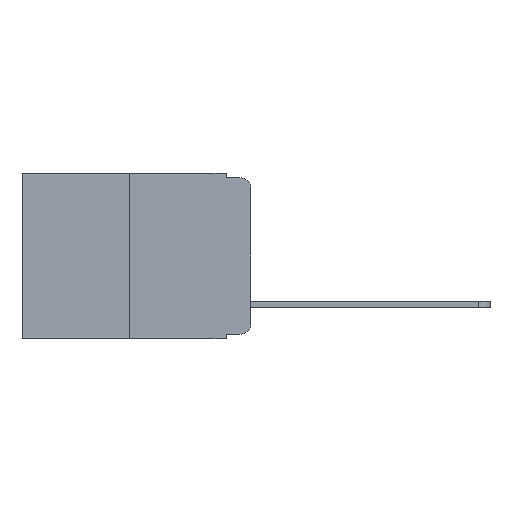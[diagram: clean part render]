
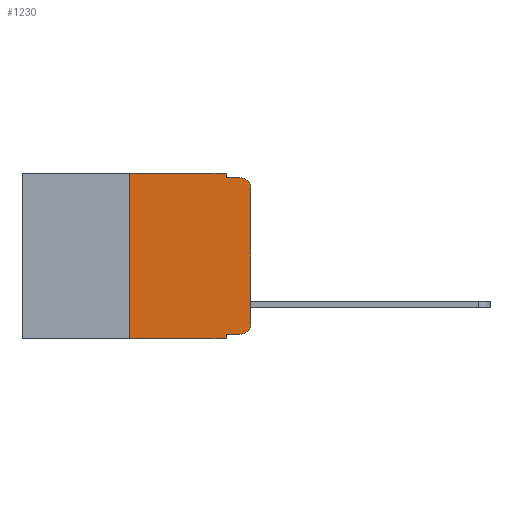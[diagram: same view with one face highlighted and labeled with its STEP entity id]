
A CAD part, left-side view. The second image highlights one B-rep face of the part: STEP entity #1230.
In plain terms, the highlighted planar face has unit normal (-1, 0, 0).
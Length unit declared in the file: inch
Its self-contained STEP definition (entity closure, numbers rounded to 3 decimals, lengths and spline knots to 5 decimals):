
#204 = CIRCLE ( 'NONE', #12012, 0.02 ) ;
#781 = CARTESIAN_POINT ( 'NONE',  ( 0., 0.02, -0.333 ) ) ;
#887 = CARTESIAN_POINT ( 'NONE',  ( 0., 0.25, 0. ) ) ;
#1215 = ORIENTED_EDGE ( 'NONE', *, *, #23683, .T. ) ;
#1230 = ADVANCED_FACE ( 'NONE', ( #8521 ), #20742, .F. ) ;
#2332 = DIRECTION ( 'NONE',  ( 0., 0., -1. ) ) ;
#2346 = VECTOR ( 'NONE', #14218, 39.37008 ) ;
#2682 = CARTESIAN_POINT ( 'NONE',  ( 0., 0.051, 0. ) ) ;
#2750 = EDGE_LOOP ( 'NONE', ( #22000, #1215, #9714, #23179, #7960, #5923, #19420, #9176, #12704, #6830 ) ) ;
#2857 = VECTOR ( 'NONE', #24087, 39.37008 ) ;
#2956 = CARTESIAN_POINT ( 'NONE',  ( 0., 0.02, -0.01 ) ) ;
#3386 = VERTEX_POINT ( 'NONE', #12868 ) ;
#3458 = EDGE_CURVE ( 'NONE', #11988, #9222, #12223, .T. ) ;
#3944 = VERTEX_POINT ( 'NONE', #2956 ) ;
#4273 = CIRCLE ( 'NONE', #19153, 0.02 ) ;
#4627 = DIRECTION ( 'NONE',  ( 0., -1., 0. ) ) ;
#4628 = DIRECTION ( 'NONE',  ( 0., -1., 0. ) ) ;
#4847 = CARTESIAN_POINT ( 'NONE',  ( 0., 0.051, -0.01 ) ) ;
#5865 = CARTESIAN_POINT ( 'NONE',  ( 0., 0.02, -0.03 ) ) ;
#5923 = ORIENTED_EDGE ( 'NONE', *, *, #20074, .F. ) ;
#5955 = CARTESIAN_POINT ( 'NONE',  ( 0., 0.25, -0.343 ) ) ;
#6243 = VERTEX_POINT ( 'NONE', #7693 ) ;
#6281 = CARTESIAN_POINT ( 'NONE',  ( 0., 0., 0. ) ) ;
#6377 = VECTOR ( 'NONE', #4628, 39.37008 ) ;
#6830 = ORIENTED_EDGE ( 'NONE', *, *, #18515, .T. ) ;
#7059 = CARTESIAN_POINT ( 'NONE',  ( 0., 0.051, -0.01 ) ) ;
#7323 = LINE ( 'NONE', #19862, #2346 ) ;
#7523 = EDGE_CURVE ( 'NONE', #9537, #10776, #7323, .T. ) ;
#7693 = CARTESIAN_POINT ( 'NONE',  ( 0., 0., -0.03 ) ) ;
#7742 = DIRECTION ( 'NONE',  ( 0., 0., -1. ) ) ;
#7840 = EDGE_CURVE ( 'NONE', #9222, #22808, #19616, .T. ) ;
#7960 = ORIENTED_EDGE ( 'NONE', *, *, #3458, .F. ) ;
#7983 = EDGE_CURVE ( 'NONE', #9537, #17198, #12288, .T. ) ;
#8521 = FACE_OUTER_BOUND ( 'NONE', #2750, .T. ) ;
#9056 = VERTEX_POINT ( 'NONE', #5955 ) ;
#9136 = CARTESIAN_POINT ( 'NONE',  ( 0., 0.051, -0.333 ) ) ;
#9176 = ORIENTED_EDGE ( 'NONE', *, *, #7523, .F. ) ;
#9222 = VERTEX_POINT ( 'NONE', #2682 ) ;
#9537 = VERTEX_POINT ( 'NONE', #9136 ) ;
#9655 = AXIS2_PLACEMENT_3D ( 'NONE', #11966, #18676, #13009 ) ;
#9714 = ORIENTED_EDGE ( 'NONE', *, *, #17434, .F. ) ;
#10776 = VERTEX_POINT ( 'NONE', #15697 ) ;
#10803 = CARTESIAN_POINT ( 'NONE',  ( 0., 0.02, -0.313 ) ) ;
#11193 = CARTESIAN_POINT ( 'NONE',  ( 0., 0.25, 0. ) ) ;
#11692 = LINE ( 'NONE', #7059, #13737 ) ;
#11705 = VECTOR ( 'NONE', #4627, 39.37008 ) ;
#11935 = EDGE_CURVE ( 'NONE', #3386, #6243, #17278, .T. ) ;
#11966 = CARTESIAN_POINT ( 'NONE',  ( 0., 0.473, 0. ) ) ;
#11988 = VERTEX_POINT ( 'NONE', #887 ) ;
#12012 = AXIS2_PLACEMENT_3D ( 'NONE', #10803, #23873, #12679 ) ;
#12223 = LINE ( 'NONE', #12339, #2857 ) ;
#12288 = LINE ( 'NONE', #17721, #11705 ) ;
#12339 = CARTESIAN_POINT ( 'NONE',  ( 0., 0.473, 0. ) ) ;
#12597 = EDGE_CURVE ( 'NONE', #9056, #10776, #16949, .T. ) ;
#12679 = DIRECTION ( 'NONE',  ( 0., 0., -1. ) ) ;
#12704 = ORIENTED_EDGE ( 'NONE', *, *, #7983, .T. ) ;
#12868 = CARTESIAN_POINT ( 'NONE',  ( 0., 0., -0.313 ) ) ;
#13009 = DIRECTION ( 'NONE',  ( 0., 0., -1. ) ) ;
#13016 = VECTOR ( 'NONE', #18785, 39.37008 ) ;
#13550 = CARTESIAN_POINT ( 'NONE',  ( 0., 0.051, 0. ) ) ;
#13737 = VECTOR ( 'NONE', #23923, 39.37008 ) ;
#14218 = DIRECTION ( 'NONE',  ( 0., 0., -1. ) ) ;
#14663 = VECTOR ( 'NONE', #2332, 39.37008 ) ;
#15697 = CARTESIAN_POINT ( 'NONE',  ( 0., 0.051, -0.343 ) ) ;
#16949 = LINE ( 'NONE', #23273, #6377 ) ;
#17198 = VERTEX_POINT ( 'NONE', #781 ) ;
#17278 = LINE ( 'NONE', #6281, #22816 ) ;
#17434 = EDGE_CURVE ( 'NONE', #22808, #3944, #11692, .T. ) ;
#17721 = CARTESIAN_POINT ( 'NONE',  ( 0., 0.051, -0.333 ) ) ;
#18515 = EDGE_CURVE ( 'NONE', #17198, #3386, #204, .T. ) ;
#18676 = DIRECTION ( 'NONE',  ( 1., 0., 0. ) ) ;
#18785 = DIRECTION ( 'NONE',  ( 0., 0., 1. ) ) ;
#18978 = DIRECTION ( 'NONE',  ( -1., 0., 0. ) ) ;
#19153 = AXIS2_PLACEMENT_3D ( 'NONE', #5865, #18978, #7742 ) ;
#19420 = ORIENTED_EDGE ( 'NONE', *, *, #12597, .T. ) ;
#19616 = LINE ( 'NONE', #13550, #14663 ) ;
#19862 = CARTESIAN_POINT ( 'NONE',  ( 0., 0.051, 0. ) ) ;
#20074 = EDGE_CURVE ( 'NONE', #9056, #11988, #22960, .T. ) ;
#20742 = PLANE ( 'NONE',  #9655 ) ;
#21272 = DIRECTION ( 'NONE',  ( 0., 0., 1. ) ) ;
#22000 = ORIENTED_EDGE ( 'NONE', *, *, #11935, .T. ) ;
#22808 = VERTEX_POINT ( 'NONE', #4847 ) ;
#22816 = VECTOR ( 'NONE', #21272, 39.37008 ) ;
#22960 = LINE ( 'NONE', #11193, #13016 ) ;
#23179 = ORIENTED_EDGE ( 'NONE', *, *, #7840, .F. ) ;
#23273 = CARTESIAN_POINT ( 'NONE',  ( 0., 0.473, -0.343 ) ) ;
#23683 = EDGE_CURVE ( 'NONE', #6243, #3944, #4273, .T. ) ;
#23873 = DIRECTION ( 'NONE',  ( -1., 0., 0. ) ) ;
#23923 = DIRECTION ( 'NONE',  ( 0., -1., 0. ) ) ;
#24087 = DIRECTION ( 'NONE',  ( 0., -1., 0. ) ) ;
